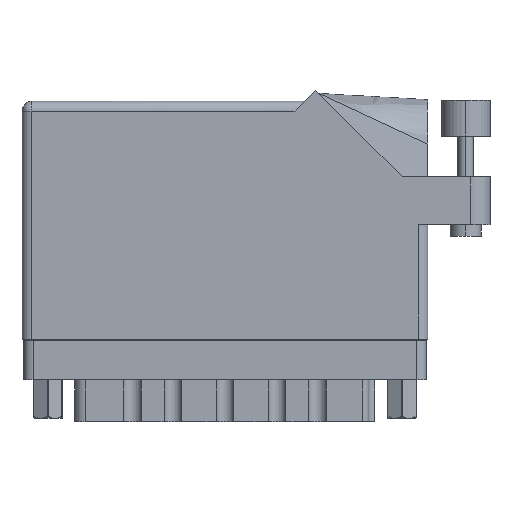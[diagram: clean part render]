
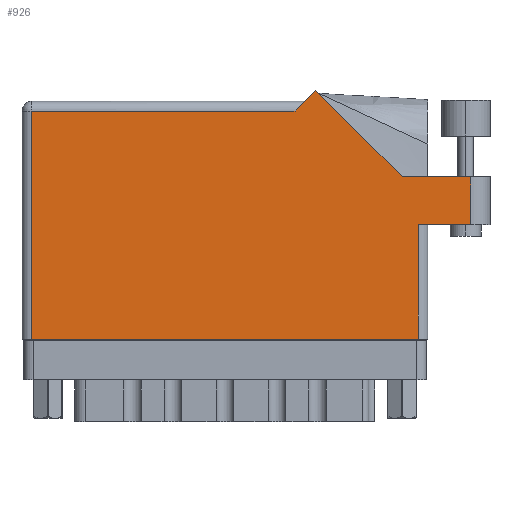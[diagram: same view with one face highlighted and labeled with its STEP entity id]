
A CAD part, front view. The second image highlights one B-rep face of the part: STEP entity #926.
In plain terms, the highlighted face is planar.
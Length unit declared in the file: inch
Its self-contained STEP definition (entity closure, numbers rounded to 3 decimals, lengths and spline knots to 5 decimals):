
#538 = LINE ( 'NONE', #56924, #5744 ) ;
#675 = VERTEX_POINT ( 'NONE', #51532 ) ;
#926 = ADVANCED_FACE ( 'NONE', ( #59637 ), #53391, .F. ) ;
#1078 = ORIENTED_EDGE ( 'NONE', *, *, #60484, .T. ) ;
#1500 = VECTOR ( 'NONE', #11842, 39.37008 ) ;
#3412 = ORIENTED_EDGE ( 'NONE', *, *, #38448, .T. ) ;
#4488 = CARTESIAN_POINT ( 'NONE',  ( 2.612, 0.737, 0. ) ) ;
#4610 = VECTOR ( 'NONE', #51783, 39.37008 ) ;
#5361 = EDGE_CURVE ( 'NONE', #40171, #29628, #538, .T. ) ;
#5744 = VECTOR ( 'NONE', #28073, 39.37008 ) ;
#7009 = VERTEX_POINT ( 'NONE', #14309 ) ;
#7608 = VECTOR ( 'NONE', #28424, 39.37008 ) ;
#8216 = VECTOR ( 'NONE', #37247, 39.37008 ) ;
#8676 = VECTOR ( 'NONE', #58754, 39.37008 ) ;
#9305 = CARTESIAN_POINT ( 'NONE',  ( 0.062, 0., 0. ) ) ;
#9856 = DIRECTION ( 'NONE',  ( -0.707, -0.707, 0. ) ) ;
#11058 = EDGE_CURVE ( 'NONE', #52566, #23484, #16096, .T. ) ;
#11842 = DIRECTION ( 'NONE',  ( 1., 0., 0. ) ) ;
#12134 = CARTESIAN_POINT ( 'NONE',  ( 2.887, 1.044, 0. ) ) ;
#12370 = DIRECTION ( 'NONE',  ( -1., 0., 0. ) ) ;
#14309 = CARTESIAN_POINT ( 'NONE',  ( 1.88971, 1.60071, 0. ) ) ;
#15008 = LINE ( 'NONE', #37043, #4610 ) ;
#16096 = LINE ( 'NONE', #4488, #53726 ) ;
#18841 = EDGE_CURVE ( 'NONE', #7009, #40171, #51863, .T. ) ;
#19031 = DIRECTION ( 'NONE',  ( 1., 0., 0. ) ) ;
#20976 = ORIENTED_EDGE ( 'NONE', *, *, #31718, .T. ) ;
#21259 = CARTESIAN_POINT ( 'NONE',  ( 0., 0., 0. ) ) ;
#22988 = CARTESIAN_POINT ( 'NONE',  ( 0.062, 1.468, 0. ) ) ;
#23379 = LINE ( 'NONE', #9305, #7608 ) ;
#23484 = VERTEX_POINT ( 'NONE', #32872 ) ;
#24540 = CARTESIAN_POINT ( 'NONE',  ( 0., 1.53, 0. ) ) ;
#25083 = CARTESIAN_POINT ( 'NONE',  ( 2.44642, 1.044, 0. ) ) ;
#27670 = CARTESIAN_POINT ( 'NONE',  ( 2.55, 0.737, 0. ) ) ;
#28073 = DIRECTION ( 'NONE',  ( -1., 0., 0. ) ) ;
#28424 = DIRECTION ( 'NONE',  ( 0., -1., 0. ) ) ;
#28704 = EDGE_LOOP ( 'NONE', ( #55914, #3412, #43769, #1078, #57974, #35653, #20976, #59022, #52204 ) ) ;
#28968 = CARTESIAN_POINT ( 'NONE',  ( 1.819, 1.53, 0. ) ) ;
#29457 = VERTEX_POINT ( 'NONE', #12134 ) ;
#29628 = VERTEX_POINT ( 'NONE', #22988 ) ;
#29951 = CARTESIAN_POINT ( 'NONE',  ( 2.55, 0., 0. ) ) ;
#31718 = EDGE_CURVE ( 'NONE', #29628, #675, #23379, .T. ) ;
#32098 = CARTESIAN_POINT ( 'NONE',  ( 2.44642, 1.044, 0. ) ) ;
#32872 = CARTESIAN_POINT ( 'NONE',  ( 2.887, 0.737, 0. ) ) ;
#34472 = VECTOR ( 'NONE', #12370, 39.37008 ) ;
#35054 = LINE ( 'NONE', #25083, #8676 ) ;
#35092 = CARTESIAN_POINT ( 'NONE',  ( 1.757, 1.468, 0. ) ) ;
#35653 = ORIENTED_EDGE ( 'NONE', *, *, #5361, .T. ) ;
#37043 = CARTESIAN_POINT ( 'NONE',  ( 2.55, 0.737, 0. ) ) ;
#37247 = DIRECTION ( 'NONE',  ( 0., 1., 0. ) ) ;
#37455 = CARTESIAN_POINT ( 'NONE',  ( 2.887, 1.044, 0. ) ) ;
#37687 = LINE ( 'NONE', #21259, #1500 ) ;
#38448 = EDGE_CURVE ( 'NONE', #23484, #29457, #56386, .T. ) ;
#38475 = EDGE_CURVE ( 'NONE', #48697, #52566, #15008, .T. ) ;
#39057 = VERTEX_POINT ( 'NONE', #32098 ) ;
#39247 = DIRECTION ( 'NONE',  ( -1., 0., 0. ) ) ;
#40171 = VERTEX_POINT ( 'NONE', #35092 ) ;
#43485 = DIRECTION ( 'NONE',  ( 0., 0., -1. ) ) ;
#43769 = ORIENTED_EDGE ( 'NONE', *, *, #56700, .T. ) ;
#44300 = LINE ( 'NONE', #46402, #34472 ) ;
#46402 = CARTESIAN_POINT ( 'NONE',  ( 3.012, 1.044, 0. ) ) ;
#48697 = VERTEX_POINT ( 'NONE', #29951 ) ;
#48820 = VECTOR ( 'NONE', #9856, 39.37008 ) ;
#51498 = EDGE_CURVE ( 'NONE', #675, #48697, #37687, .T. ) ;
#51532 = CARTESIAN_POINT ( 'NONE',  ( 0.062, 0., 0. ) ) ;
#51783 = DIRECTION ( 'NONE',  ( 0., 1., 0. ) ) ;
#51863 = LINE ( 'NONE', #28968, #48820 ) ;
#52204 = ORIENTED_EDGE ( 'NONE', *, *, #38475, .T. ) ;
#52566 = VERTEX_POINT ( 'NONE', #27670 ) ;
#53391 = PLANE ( 'NONE',  #54619 ) ;
#53726 = VECTOR ( 'NONE', #19031, 39.37008 ) ;
#54619 = AXIS2_PLACEMENT_3D ( 'NONE', #24540, #43485, #39247 ) ;
#55914 = ORIENTED_EDGE ( 'NONE', *, *, #11058, .T. ) ;
#56386 = LINE ( 'NONE', #37455, #8216 ) ;
#56700 = EDGE_CURVE ( 'NONE', #29457, #39057, #44300, .T. ) ;
#56924 = CARTESIAN_POINT ( 'NONE',  ( 0., 1.468, 0. ) ) ;
#57974 = ORIENTED_EDGE ( 'NONE', *, *, #18841, .T. ) ;
#58754 = DIRECTION ( 'NONE',  ( -0.707, 0.707, 0. ) ) ;
#59022 = ORIENTED_EDGE ( 'NONE', *, *, #51498, .T. ) ;
#59637 = FACE_OUTER_BOUND ( 'NONE', #28704, .T. ) ;
#60484 = EDGE_CURVE ( 'NONE', #39057, #7009, #35054, .T. ) ;
